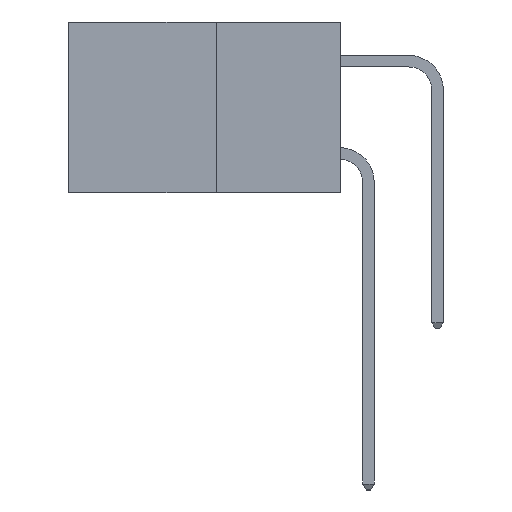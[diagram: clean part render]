
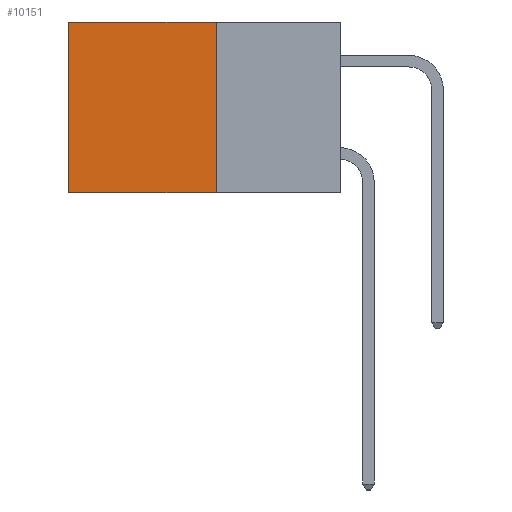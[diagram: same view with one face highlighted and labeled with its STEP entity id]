
A CAD part, left-side view. The second image highlights one B-rep face of the part: STEP entity #10151.
In plain terms, the highlighted planar face has unit normal (-1, 0, 0).
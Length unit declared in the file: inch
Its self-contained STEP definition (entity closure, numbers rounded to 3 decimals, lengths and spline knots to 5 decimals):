
#102 = DIRECTION ( 'NONE',  ( 0., 0., -1. ) ) ;
#155 = CARTESIAN_POINT ( 'NONE',  ( 0.277, 0.27, -0.37 ) ) ;
#194 = LINE ( 'NONE', #11888, #5041 ) ;
#276 = VERTEX_POINT ( 'NONE', #809 ) ;
#565 = EDGE_CURVE ( 'NONE', #3105, #709, #194, .T. ) ;
#658 = CARTESIAN_POINT ( 'NONE',  ( 0.277, 0.27, -0.37 ) ) ;
#709 = VERTEX_POINT ( 'NONE', #1471 ) ;
#809 = CARTESIAN_POINT ( 'NONE',  ( 0.277, 0.27, -0.37 ) ) ;
#1294 = VERTEX_POINT ( 'NONE', #7070 ) ;
#1471 = CARTESIAN_POINT ( 'NONE',  ( 0.277, 0.59, -0.37 ) ) ;
#1520 = VECTOR ( 'NONE', #8597, 39.37008 ) ;
#2317 = LINE ( 'NONE', #155, #9405 ) ;
#3105 = VERTEX_POINT ( 'NONE', #6201 ) ;
#3775 = CARTESIAN_POINT ( 'NONE',  ( 0.277, 0.27, -0.37 ) ) ;
#4566 = DIRECTION ( 'NONE',  ( 0., 0., -1. ) ) ;
#4893 = CARTESIAN_POINT ( 'NONE',  ( 0.277, 0.27, 0. ) ) ;
#5041 = VECTOR ( 'NONE', #102, 39.37008 ) ;
#5433 = ORIENTED_EDGE ( 'NONE', *, *, #565, .T. ) ;
#5631 = EDGE_CURVE ( 'NONE', #276, #709, #2317, .T. ) ;
#5881 = DIRECTION ( 'NONE',  ( 0., 1., 0. ) ) ;
#5964 = LINE ( 'NONE', #4893, #11033 ) ;
#6166 = ORIENTED_EDGE ( 'NONE', *, *, #5631, .F. ) ;
#6201 = CARTESIAN_POINT ( 'NONE',  ( 0.277, 0.59, 0. ) ) ;
#6480 = ORIENTED_EDGE ( 'NONE', *, *, #10269, .F. ) ;
#6702 = LINE ( 'NONE', #3775, #1520 ) ;
#7034 = AXIS2_PLACEMENT_3D ( 'NONE', #658, #10340, #4566 ) ;
#7070 = CARTESIAN_POINT ( 'NONE',  ( 0.277, 0.27, 0. ) ) ;
#7228 = ORIENTED_EDGE ( 'NONE', *, *, #9165, .T. ) ;
#8597 = DIRECTION ( 'NONE',  ( 0., 0., -1. ) ) ;
#9165 = EDGE_CURVE ( 'NONE', #1294, #3105, #5964, .T. ) ;
#9405 = VECTOR ( 'NONE', #12365, 39.37008 ) ;
#10151 = ADVANCED_FACE ( 'NONE', ( #10733 ), #10296, .F. ) ;
#10269 = EDGE_CURVE ( 'NONE', #1294, #276, #6702, .T. ) ;
#10296 = PLANE ( 'NONE',  #7034 ) ;
#10340 = DIRECTION ( 'NONE',  ( 1., 0., 0. ) ) ;
#10733 = FACE_OUTER_BOUND ( 'NONE', #11851, .T. ) ;
#11033 = VECTOR ( 'NONE', #5881, 39.37008 ) ;
#11851 = EDGE_LOOP ( 'NONE', ( #5433, #6166, #6480, #7228 ) ) ;
#11888 = CARTESIAN_POINT ( 'NONE',  ( 0.277, 0.59, -0.37 ) ) ;
#12365 = DIRECTION ( 'NONE',  ( 0., 1., 0. ) ) ;
